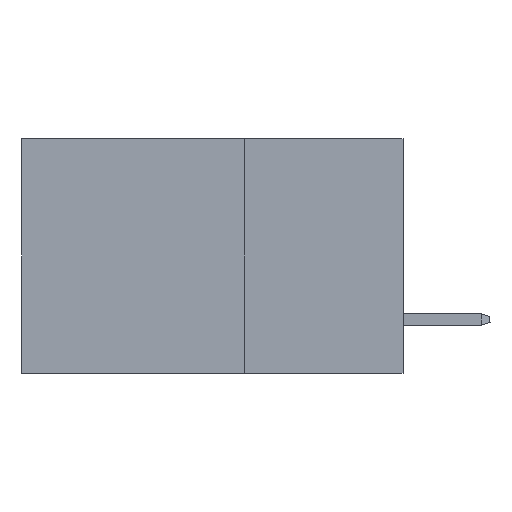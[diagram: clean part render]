
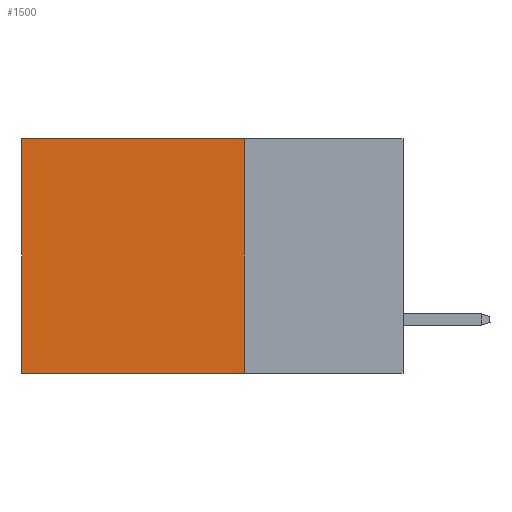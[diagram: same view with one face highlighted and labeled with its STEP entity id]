
A CAD part, left-side view. The second image highlights one B-rep face of the part: STEP entity #1500.
In plain terms, the highlighted planar face has unit normal (-1, 0, 0).
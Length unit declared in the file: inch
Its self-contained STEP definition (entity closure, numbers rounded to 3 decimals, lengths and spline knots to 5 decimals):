
#661 = ORIENTED_EDGE ( 'NONE', *, *, #15230, .T. ) ;
#822 = FACE_OUTER_BOUND ( 'NONE', #17636, .T. ) ;
#1252 = LINE ( 'NONE', #30735, #18467 ) ;
#1379 = EDGE_CURVE ( 'NONE', #27536, #22187, #10425, .T. ) ;
#1500 = ADVANCED_FACE ( 'NONE', ( #822 ), #8175, .F. ) ;
#3784 = ORIENTED_EDGE ( 'NONE', *, *, #13970, .F. ) ;
#3903 = LINE ( 'NONE', #18458, #22205 ) ;
#5787 = DIRECTION ( 'NONE',  ( 0., 0., -1. ) ) ;
#6734 = VECTOR ( 'NONE', #14627, 39.37008 ) ;
#7259 = LINE ( 'NONE', #29551, #6734 ) ;
#8175 = PLANE ( 'NONE',  #9174 ) ;
#8309 = EDGE_CURVE ( 'NONE', #27536, #9010, #3903, .T. ) ;
#8605 = VERTEX_POINT ( 'NONE', #12671 ) ;
#8606 = DIRECTION ( 'NONE',  ( 0., 0., -1. ) ) ;
#9010 = VERTEX_POINT ( 'NONE', #20796 ) ;
#9174 = AXIS2_PLACEMENT_3D ( 'NONE', #17940, #27733, #5787 ) ;
#10425 = LINE ( 'NONE', #23097, #24542 ) ;
#12671 = CARTESIAN_POINT ( 'NONE',  ( 0.2875, 0.6, -0.37 ) ) ;
#13970 = EDGE_CURVE ( 'NONE', #22187, #8605, #7259, .T. ) ;
#14627 = DIRECTION ( 'NONE',  ( 0., 1., 0. ) ) ;
#15230 = EDGE_CURVE ( 'NONE', #9010, #8605, #1252, .T. ) ;
#15523 = CARTESIAN_POINT ( 'NONE',  ( 0.2875, 0.25, 0. ) ) ;
#15699 = DIRECTION ( 'NONE',  ( 0., 0., -1. ) ) ;
#17636 = EDGE_LOOP ( 'NONE', ( #661, #3784, #29298, #23110 ) ) ;
#17940 = CARTESIAN_POINT ( 'NONE',  ( 0.2875, 0.25, 0. ) ) ;
#18458 = CARTESIAN_POINT ( 'NONE',  ( 0.2875, 0.25, 0. ) ) ;
#18467 = VECTOR ( 'NONE', #8606, 39.37008 ) ;
#20796 = CARTESIAN_POINT ( 'NONE',  ( 0.2875, 0.6, 0. ) ) ;
#22187 = VERTEX_POINT ( 'NONE', #22676 ) ;
#22205 = VECTOR ( 'NONE', #28242, 39.37008 ) ;
#22676 = CARTESIAN_POINT ( 'NONE',  ( 0.2875, 0.25, -0.37 ) ) ;
#23097 = CARTESIAN_POINT ( 'NONE',  ( 0.2875, 0.25, 0. ) ) ;
#23110 = ORIENTED_EDGE ( 'NONE', *, *, #8309, .T. ) ;
#24542 = VECTOR ( 'NONE', #15699, 39.37008 ) ;
#27536 = VERTEX_POINT ( 'NONE', #15523 ) ;
#27733 = DIRECTION ( 'NONE',  ( 1., 0., 0. ) ) ;
#28242 = DIRECTION ( 'NONE',  ( 0., 1., 0. ) ) ;
#29298 = ORIENTED_EDGE ( 'NONE', *, *, #1379, .F. ) ;
#29551 = CARTESIAN_POINT ( 'NONE',  ( 0.2875, 0.25, -0.37 ) ) ;
#30735 = CARTESIAN_POINT ( 'NONE',  ( 0.2875, 0.6, 0. ) ) ;
